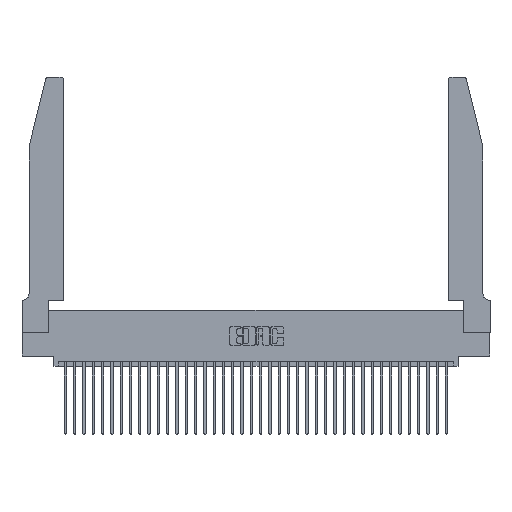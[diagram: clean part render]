
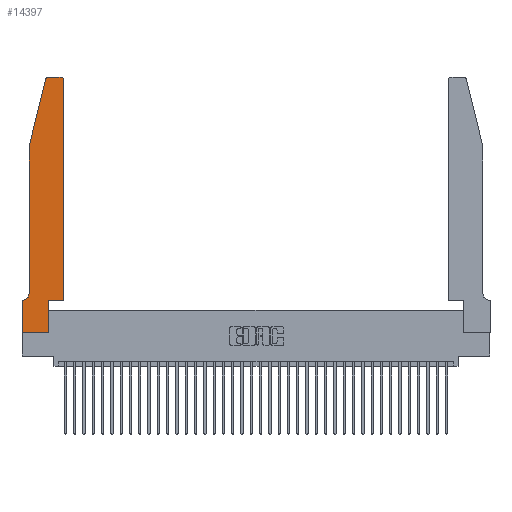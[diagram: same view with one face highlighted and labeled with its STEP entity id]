
A CAD part, top view. The second image highlights one B-rep face of the part: STEP entity #14397.
In plain terms, the highlighted planar face has unit normal (0, 0, 1).
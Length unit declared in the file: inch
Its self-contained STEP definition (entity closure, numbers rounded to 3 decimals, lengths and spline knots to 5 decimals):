
#380 = EDGE_CURVE ( 'NONE', #15649, #15787, #10668, .T. ) ;
#1190 = LINE ( 'NONE', #25247, #19529 ) ;
#2354 = ORIENTED_EDGE ( 'NONE', *, *, #31838, .T. ) ;
#2526 = CARTESIAN_POINT ( 'NONE',  ( 0.4505, 0.35, 0.37 ) ) ;
#3092 = DIRECTION ( 'NONE',  ( -1., 0., 0. ) ) ;
#3285 = AXIS2_PLACEMENT_3D ( 'NONE', #33946, #14499, #5290 ) ;
#3348 = CARTESIAN_POINT ( 'NONE',  ( 0.4205, 2.75, 0.37 ) ) ;
#4913 = EDGE_LOOP ( 'NONE', ( #18166, #15004, #36919, #31125, #6764, #35142, #15735, #7241, #9008, #16781, #8440, #2354 ) ) ;
#5001 = DIRECTION ( 'NONE',  ( 1., 0., 0. ) ) ;
#5290 = DIRECTION ( 'NONE',  ( 1., 0., 0. ) ) ;
#5459 = LINE ( 'NONE', #11227, #37052 ) ;
#5941 = CARTESIAN_POINT ( 'NONE',  ( 0., 0.35, 0.37 ) ) ;
#6152 = CARTESIAN_POINT ( 'NONE',  ( 0.0755, 2., 0.37 ) ) ;
#6331 = CARTESIAN_POINT ( 'NONE',  ( 0.4505, 2.72, 0.37 ) ) ;
#6764 = ORIENTED_EDGE ( 'NONE', *, *, #25897, .T. ) ;
#7241 = ORIENTED_EDGE ( 'NONE', *, *, #19329, .T. ) ;
#8440 = ORIENTED_EDGE ( 'NONE', *, *, #34379, .T. ) ;
#9008 = ORIENTED_EDGE ( 'NONE', *, *, #18638, .T. ) ;
#9196 = CARTESIAN_POINT ( 'NONE',  ( 0.25487, 2.72718, 0.37 ) ) ;
#9346 = VERTEX_POINT ( 'NONE', #2526 ) ;
#9467 = VECTOR ( 'NONE', #23292, 39.37008 ) ;
#9530 = CARTESIAN_POINT ( 'NONE',  ( 0.0755, 2., 0.37 ) ) ;
#9616 = CARTESIAN_POINT ( 'NONE',  ( 0., 0., 0.37 ) ) ;
#10038 = VECTOR ( 'NONE', #25876, 39.37008 ) ;
#10668 = LINE ( 'NONE', #28497, #29842 ) ;
#10878 = FACE_OUTER_BOUND ( 'NONE', #4913, .T. ) ;
#11227 = CARTESIAN_POINT ( 'NONE',  ( 0.4505, 0.35, 0.37 ) ) ;
#13060 = DIRECTION ( 'NONE',  ( -1., 0., 0. ) ) ;
#13170 = DIRECTION ( 'NONE',  ( 0., -1., 0. ) ) ;
#14397 = ADVANCED_FACE ( 'NONE', ( #10878 ), #25616, .T. ) ;
#14499 = DIRECTION ( 'NONE',  ( 0., 0., 1. ) ) ;
#15004 = ORIENTED_EDGE ( 'NONE', *, *, #25286, .T. ) ;
#15649 = VERTEX_POINT ( 'NONE', #3348 ) ;
#15678 = AXIS2_PLACEMENT_3D ( 'NONE', #36325, #30141, #13060 ) ;
#15735 = ORIENTED_EDGE ( 'NONE', *, *, #22766, .T. ) ;
#15787 = VERTEX_POINT ( 'NONE', #20921 ) ;
#16781 = ORIENTED_EDGE ( 'NONE', *, *, #36485, .T. ) ;
#16794 = DIRECTION ( 'NONE',  ( 1., 0., 0. ) ) ;
#17016 = VERTEX_POINT ( 'NONE', #22230 ) ;
#17754 = CARTESIAN_POINT ( 'NONE',  ( 0.0755, 0.42, 0.37 ) ) ;
#17815 = VECTOR ( 'NONE', #3092, 39.37008 ) ;
#18029 = EDGE_CURVE ( 'NONE', #18934, #19910, #26592, .T. ) ;
#18166 = ORIENTED_EDGE ( 'NONE', *, *, #380, .T. ) ;
#18278 = CARTESIAN_POINT ( 'NONE',  ( 0.2865, 0.35, 0.37 ) ) ;
#18638 = EDGE_CURVE ( 'NONE', #17016, #25791, #24659, .T. ) ;
#18760 = EDGE_CURVE ( 'NONE', #35430, #20455, #25614, .T. ) ;
#18934 = VERTEX_POINT ( 'NONE', #31612 ) ;
#19329 = EDGE_CURVE ( 'NONE', #20608, #17016, #37097, .T. ) ;
#19529 = VECTOR ( 'NONE', #28309, 39.37008 ) ;
#19601 = CARTESIAN_POINT ( 'NONE',  ( 0., 0., 0.37 ) ) ;
#19910 = VERTEX_POINT ( 'NONE', #17754 ) ;
#20455 = VERTEX_POINT ( 'NONE', #5941 ) ;
#20485 = CARTESIAN_POINT ( 'NONE',  ( 0.2865, 0.35, 0.37 ) ) ;
#20608 = VERTEX_POINT ( 'NONE', #9616 ) ;
#20921 = CARTESIAN_POINT ( 'NONE',  ( 0.284, 2.75, 0.37 ) ) ;
#21077 = VECTOR ( 'NONE', #26809, 39.37008 ) ;
#21396 = CARTESIAN_POINT ( 'NONE',  ( 0.284, 2.72, 0.37 ) ) ;
#21979 = VECTOR ( 'NONE', #16794, 39.37008 ) ;
#22230 = CARTESIAN_POINT ( 'NONE',  ( 0.2865, 0., 0.37 ) ) ;
#22357 = CARTESIAN_POINT ( 'NONE',  ( 0.0055, 0.35, 0.37 ) ) ;
#22534 = VERTEX_POINT ( 'NONE', #9196 ) ;
#22540 = DIRECTION ( 'NONE',  ( 0., 0., 1. ) ) ;
#22766 = EDGE_CURVE ( 'NONE', #20455, #20608, #27927, .T. ) ;
#23217 = VERTEX_POINT ( 'NONE', #6331 ) ;
#23292 = DIRECTION ( 'NONE',  ( -0.239, -0.971, 0. ) ) ;
#24403 = EDGE_CURVE ( 'NONE', #22534, #18934, #26444, .T. ) ;
#24659 = LINE ( 'NONE', #20485, #10038 ) ;
#24732 = VECTOR ( 'NONE', #13170, 39.37008 ) ;
#25247 = CARTESIAN_POINT ( 'NONE',  ( 0.4505, 0.35, 0.37 ) ) ;
#25286 = EDGE_CURVE ( 'NONE', #15787, #22534, #32786, .T. ) ;
#25614 = LINE ( 'NONE', #32631, #17815 ) ;
#25616 = PLANE ( 'NONE',  #3285 ) ;
#25791 = VERTEX_POINT ( 'NONE', #18278 ) ;
#25876 = DIRECTION ( 'NONE',  ( 0., 1., 0. ) ) ;
#25897 = EDGE_CURVE ( 'NONE', #19910, #35430, #26342, .T. ) ;
#26342 = CIRCLE ( 'NONE', #15678, 0.07 ) ;
#26444 = LINE ( 'NONE', #6152, #9467 ) ;
#26592 = LINE ( 'NONE', #9530, #21077 ) ;
#26809 = DIRECTION ( 'NONE',  ( 0., -1., 0. ) ) ;
#27285 = DIRECTION ( 'NONE',  ( -1., 0., 0. ) ) ;
#27927 = LINE ( 'NONE', #36944, #24732 ) ;
#28309 = DIRECTION ( 'NONE',  ( 1., 0., 0. ) ) ;
#28497 = CARTESIAN_POINT ( 'NONE',  ( 0.2605, 2.75, 0.37 ) ) ;
#28883 = AXIS2_PLACEMENT_3D ( 'NONE', #21396, #32796, #33294 ) ;
#29842 = VECTOR ( 'NONE', #27285, 39.37008 ) ;
#30141 = DIRECTION ( 'NONE',  ( 0., 0., -1. ) ) ;
#30185 = AXIS2_PLACEMENT_3D ( 'NONE', #34425, #22540, #5001 ) ;
#31125 = ORIENTED_EDGE ( 'NONE', *, *, #18029, .T. ) ;
#31612 = CARTESIAN_POINT ( 'NONE',  ( 0.0755, 2., 0.37 ) ) ;
#31838 = EDGE_CURVE ( 'NONE', #23217, #15649, #34381, .T. ) ;
#32631 = CARTESIAN_POINT ( 'NONE',  ( 0.0755, 0.35, 0.37 ) ) ;
#32786 = CIRCLE ( 'NONE', #28883, 0.03 ) ;
#32796 = DIRECTION ( 'NONE',  ( 0., 0., 1. ) ) ;
#33294 = DIRECTION ( 'NONE',  ( 1., 0., 0. ) ) ;
#33946 = CARTESIAN_POINT ( 'NONE',  ( 0., 0.35, 0.37 ) ) ;
#34379 = EDGE_CURVE ( 'NONE', #9346, #23217, #5459, .T. ) ;
#34381 = CIRCLE ( 'NONE', #30185, 0.03 ) ;
#34425 = CARTESIAN_POINT ( 'NONE',  ( 0.4205, 2.72, 0.37 ) ) ;
#34853 = DIRECTION ( 'NONE',  ( 0., 1., 0. ) ) ;
#35142 = ORIENTED_EDGE ( 'NONE', *, *, #18760, .T. ) ;
#35430 = VERTEX_POINT ( 'NONE', #22357 ) ;
#36325 = CARTESIAN_POINT ( 'NONE',  ( 0.0055, 0.42, 0.37 ) ) ;
#36485 = EDGE_CURVE ( 'NONE', #25791, #9346, #1190, .T. ) ;
#36919 = ORIENTED_EDGE ( 'NONE', *, *, #24403, .T. ) ;
#36944 = CARTESIAN_POINT ( 'NONE',  ( 0., 0., 0.37 ) ) ;
#37052 = VECTOR ( 'NONE', #34853, 39.37008 ) ;
#37097 = LINE ( 'NONE', #19601, #21979 ) ;
